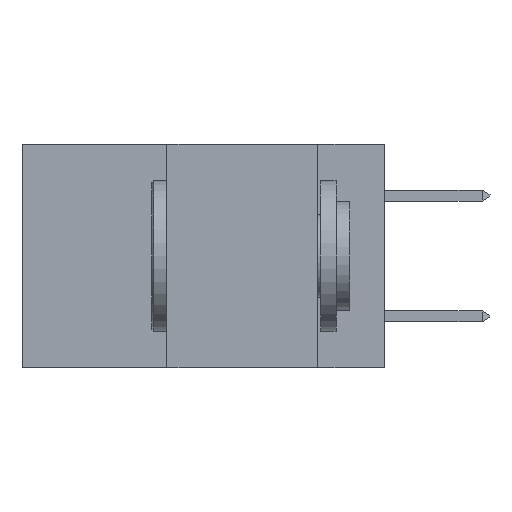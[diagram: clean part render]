
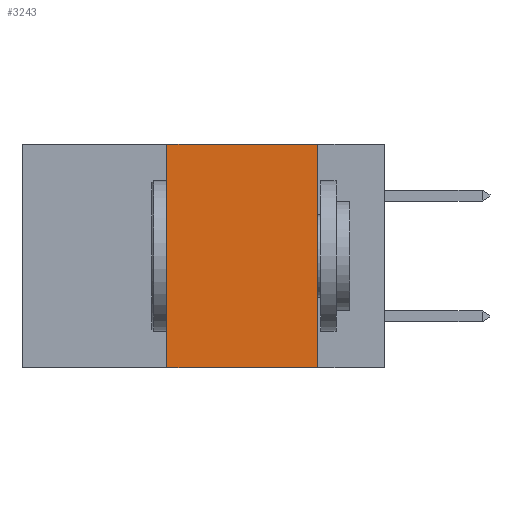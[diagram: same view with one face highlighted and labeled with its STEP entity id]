
A CAD part, left-side view. The second image highlights one B-rep face of the part: STEP entity #3243.
In plain terms, the highlighted planar face has unit normal (-1, 0, 0).
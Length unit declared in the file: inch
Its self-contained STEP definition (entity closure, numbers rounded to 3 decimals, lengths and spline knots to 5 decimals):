
#42 = LINE ( 'NONE', #12963, #8445 ) ;
#413 = EDGE_LOOP ( 'NONE', ( #8765, #12151, #14054, #2279 ) ) ;
#774 = VECTOR ( 'NONE', #13610, 39.37008 ) ;
#1273 = VERTEX_POINT ( 'NONE', #3754 ) ;
#1791 = FACE_OUTER_BOUND ( 'NONE', #413, .T. ) ;
#2279 = ORIENTED_EDGE ( 'NONE', *, *, #13301, .T. ) ;
#2450 = EDGE_CURVE ( 'NONE', #15978, #4459, #16148, .T. ) ;
#2785 = DIRECTION ( 'NONE',  ( 0., 0., -1. ) ) ;
#2883 = VECTOR ( 'NONE', #8405, 39.37008 ) ;
#3243 = ADVANCED_FACE ( 'NONE', ( #1791 ), #7909, .F. ) ;
#3754 = CARTESIAN_POINT ( 'NONE',  ( 0., 0.36, 0. ) ) ;
#4459 = VERTEX_POINT ( 'NONE', #8246 ) ;
#5372 = DIRECTION ( 'NONE',  ( 1., 0., 0. ) ) ;
#6465 = DIRECTION ( 'NONE',  ( 0., -1., 0. ) ) ;
#7754 = LINE ( 'NONE', #11655, #11650 ) ;
#7909 = PLANE ( 'NONE',  #12617 ) ;
#8080 = CARTESIAN_POINT ( 'NONE',  ( 0., 0.11, 0. ) ) ;
#8246 = CARTESIAN_POINT ( 'NONE',  ( 0., 0.11, -0.37 ) ) ;
#8405 = DIRECTION ( 'NONE',  ( 0., -1., 0. ) ) ;
#8445 = VECTOR ( 'NONE', #8850, 39.37008 ) ;
#8765 = ORIENTED_EDGE ( 'NONE', *, *, #2450, .F. ) ;
#8850 = DIRECTION ( 'NONE',  ( 0., 0., 1. ) ) ;
#8918 = EDGE_CURVE ( 'NONE', #12059, #1273, #42, .T. ) ;
#10542 = CARTESIAN_POINT ( 'NONE',  ( 0., 0.6, 0. ) ) ;
#11650 = VECTOR ( 'NONE', #6465, 39.37008 ) ;
#11655 = CARTESIAN_POINT ( 'NONE',  ( 0., 0.6, -0.37 ) ) ;
#12059 = VERTEX_POINT ( 'NONE', #16907 ) ;
#12151 = ORIENTED_EDGE ( 'NONE', *, *, #16827, .F. ) ;
#12293 = CARTESIAN_POINT ( 'NONE',  ( 0., 0.11, 0. ) ) ;
#12617 = AXIS2_PLACEMENT_3D ( 'NONE', #10542, #5372, #2785 ) ;
#12963 = CARTESIAN_POINT ( 'NONE',  ( 0., 0.36, 0. ) ) ;
#13301 = EDGE_CURVE ( 'NONE', #12059, #4459, #7754, .T. ) ;
#13610 = DIRECTION ( 'NONE',  ( 0., 0., -1. ) ) ;
#13983 = LINE ( 'NONE', #15768, #2883 ) ;
#14054 = ORIENTED_EDGE ( 'NONE', *, *, #8918, .F. ) ;
#15768 = CARTESIAN_POINT ( 'NONE',  ( 0., 0.6, 0. ) ) ;
#15978 = VERTEX_POINT ( 'NONE', #8080 ) ;
#16148 = LINE ( 'NONE', #12293, #774 ) ;
#16827 = EDGE_CURVE ( 'NONE', #1273, #15978, #13983, .T. ) ;
#16907 = CARTESIAN_POINT ( 'NONE',  ( 0., 0.36, -0.37 ) ) ;
